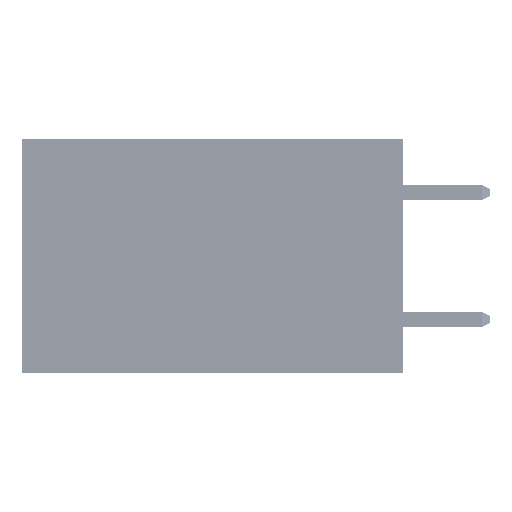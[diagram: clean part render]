
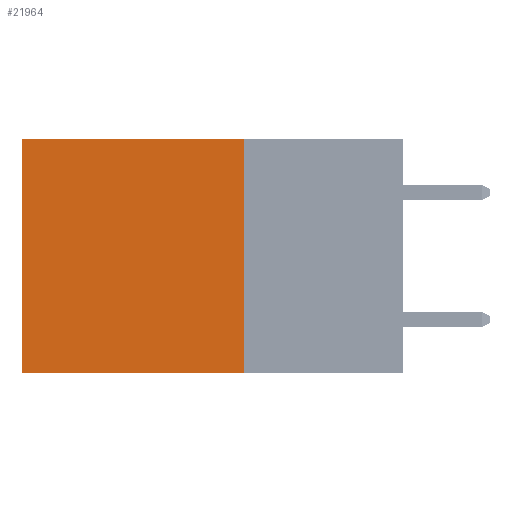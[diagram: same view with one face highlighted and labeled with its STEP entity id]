
A CAD part, left-side view. The second image highlights one B-rep face of the part: STEP entity #21964.
In plain terms, the highlighted planar face has unit normal (-1, 0, 0).
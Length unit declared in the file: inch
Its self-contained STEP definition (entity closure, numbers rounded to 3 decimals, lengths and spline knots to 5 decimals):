
#852 = VERTEX_POINT ( 'NONE', #26923 ) ;
#953 = DIRECTION ( 'NONE',  ( 1., 0., 0. ) ) ;
#2634 = ORIENTED_EDGE ( 'NONE', *, *, #25489, .T. ) ;
#4548 = VERTEX_POINT ( 'NONE', #32599 ) ;
#5802 = LINE ( 'NONE', #39742, #14086 ) ;
#8302 = EDGE_CURVE ( 'NONE', #852, #4548, #25642, .T. ) ;
#9845 = CARTESIAN_POINT ( 'NONE',  ( 0.2875, 0.6, -0.37 ) ) ;
#9962 = DIRECTION ( 'NONE',  ( 0., 0., -1. ) ) ;
#11780 = DIRECTION ( 'NONE',  ( 0., 1., 0. ) ) ;
#12284 = ORIENTED_EDGE ( 'NONE', *, *, #33540, .F. ) ;
#12571 = VECTOR ( 'NONE', #11780, 39.37008 ) ;
#12861 = CARTESIAN_POINT ( 'NONE',  ( 0.2875, 0.25, 0. ) ) ;
#14086 = VECTOR ( 'NONE', #15794, 39.37008 ) ;
#14905 = AXIS2_PLACEMENT_3D ( 'NONE', #12861, #953, #37001 ) ;
#15794 = DIRECTION ( 'NONE',  ( 0., 0., -1. ) ) ;
#16481 = ORIENTED_EDGE ( 'NONE', *, *, #8302, .F. ) ;
#18815 = CARTESIAN_POINT ( 'NONE',  ( 0.2875, 0.6, 0. ) ) ;
#21964 = ADVANCED_FACE ( 'NONE', ( #24024 ), #44944, .F. ) ;
#23172 = VECTOR ( 'NONE', #23511, 39.37008 ) ;
#23511 = DIRECTION ( 'NONE',  ( 0., 1., 0. ) ) ;
#24024 = FACE_OUTER_BOUND ( 'NONE', #45160, .T. ) ;
#25489 = EDGE_CURVE ( 'NONE', #28687, #27713, #5802, .T. ) ;
#25642 = LINE ( 'NONE', #41872, #33889 ) ;
#26923 = CARTESIAN_POINT ( 'NONE',  ( 0.2875, 0.25, 0. ) ) ;
#27393 = ORIENTED_EDGE ( 'NONE', *, *, #48558, .T. ) ;
#27713 = VERTEX_POINT ( 'NONE', #9845 ) ;
#27761 = CARTESIAN_POINT ( 'NONE',  ( 0.2875, 0.25, -0.37 ) ) ;
#28257 = LINE ( 'NONE', #43337, #23172 ) ;
#28687 = VERTEX_POINT ( 'NONE', #18815 ) ;
#32599 = CARTESIAN_POINT ( 'NONE',  ( 0.2875, 0.25, -0.37 ) ) ;
#33540 = EDGE_CURVE ( 'NONE', #4548, #27713, #51251, .T. ) ;
#33889 = VECTOR ( 'NONE', #9962, 39.37008 ) ;
#37001 = DIRECTION ( 'NONE',  ( 0., 0., -1. ) ) ;
#39742 = CARTESIAN_POINT ( 'NONE',  ( 0.2875, 0.6, 0. ) ) ;
#41872 = CARTESIAN_POINT ( 'NONE',  ( 0.2875, 0.25, 0. ) ) ;
#43337 = CARTESIAN_POINT ( 'NONE',  ( 0.2875, 0.25, 0. ) ) ;
#44944 = PLANE ( 'NONE',  #14905 ) ;
#45160 = EDGE_LOOP ( 'NONE', ( #2634, #12284, #16481, #27393 ) ) ;
#48558 = EDGE_CURVE ( 'NONE', #852, #28687, #28257, .T. ) ;
#51251 = LINE ( 'NONE', #27761, #12571 ) ;
